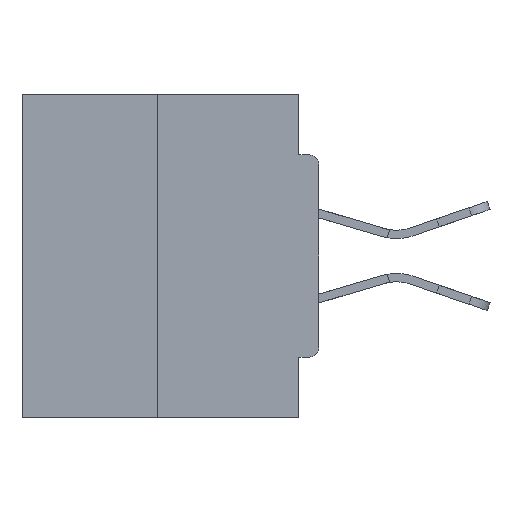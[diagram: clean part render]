
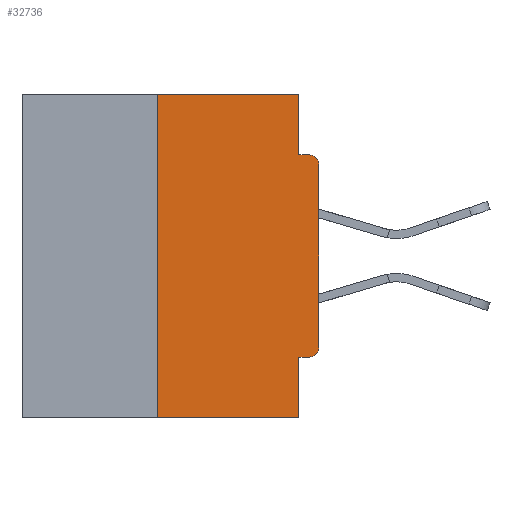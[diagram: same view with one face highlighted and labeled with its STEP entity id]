
A CAD part, left-side view. The second image highlights one B-rep face of the part: STEP entity #32736.
In plain terms, the highlighted planar face has unit normal (-1, 0, 0).
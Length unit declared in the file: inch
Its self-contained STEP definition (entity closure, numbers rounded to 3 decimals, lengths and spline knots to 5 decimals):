
#565 = CARTESIAN_POINT ( 'NONE',  ( 0., 0.25, 0. ) ) ;
#1227 = LINE ( 'NONE', #565, #5970 ) ;
#1453 = CARTESIAN_POINT ( 'NONE',  ( 0., 0.031, -0.0935 ) ) ;
#1588 = DIRECTION ( 'NONE',  ( -1., 0., 0. ) ) ;
#1603 = CARTESIAN_POINT ( 'NONE',  ( 0., 0., -0.3915 ) ) ;
#2099 = CARTESIAN_POINT ( 'NONE',  ( 0., 0.015, -0.0935 ) ) ;
#2642 = CARTESIAN_POINT ( 'NONE',  ( 0., 0., -0.4065 ) ) ;
#2885 = DIRECTION ( 'NONE',  ( 0., 1., 0. ) ) ;
#3850 = DIRECTION ( 'NONE',  ( 0., -1., 0. ) ) ;
#4548 = DIRECTION ( 'NONE',  ( -1., 0., 0. ) ) ;
#5272 = EDGE_CURVE ( 'NONE', #11194, #31900, #14237, .T. ) ;
#5275 = LINE ( 'NONE', #2642, #33623 ) ;
#5970 = VECTOR ( 'NONE', #25760, 39.37008 ) ;
#6230 = EDGE_CURVE ( 'NONE', #16097, #21846, #12427, .T. ) ;
#6483 = EDGE_CURVE ( 'NONE', #30119, #7789, #28742, .T. ) ;
#6925 = VECTOR ( 'NONE', #12689, 39.37008 ) ;
#7132 = LINE ( 'NONE', #23174, #15722 ) ;
#7213 = CARTESIAN_POINT ( 'NONE',  ( 0., 0.46, 0. ) ) ;
#7335 = DIRECTION ( 'NONE',  ( 0., 0., -1. ) ) ;
#7745 = ORIENTED_EDGE ( 'NONE', *, *, #12949, .F. ) ;
#7789 = VERTEX_POINT ( 'NONE', #22108 ) ;
#7847 = DIRECTION ( 'NONE',  ( 0., 0., 1. ) ) ;
#8564 = VECTOR ( 'NONE', #11351, 39.37008 ) ;
#8926 = CARTESIAN_POINT ( 'NONE',  ( 0., 0.46, 0. ) ) ;
#10336 = EDGE_CURVE ( 'NONE', #16097, #30119, #5275, .T. ) ;
#11194 = VERTEX_POINT ( 'NONE', #1453 ) ;
#11351 = DIRECTION ( 'NONE',  ( 0., 0., -1. ) ) ;
#12427 = CIRCLE ( 'NONE', #19663, 0.015 ) ;
#12654 = CARTESIAN_POINT ( 'NONE',  ( 0., 0.015, -0.1085 ) ) ;
#12689 = DIRECTION ( 'NONE',  ( 0., -1., 0. ) ) ;
#12803 = CARTESIAN_POINT ( 'NONE',  ( 0., 0., -0.0935 ) ) ;
#12949 = EDGE_CURVE ( 'NONE', #30383, #27522, #1227, .T. ) ;
#13443 = DIRECTION ( 'NONE',  ( 0., 0., -1. ) ) ;
#13752 = FACE_OUTER_BOUND ( 'NONE', #21500, .T. ) ;
#14123 = ORIENTED_EDGE ( 'NONE', *, *, #6230, .T. ) ;
#14237 = LINE ( 'NONE', #12803, #6925 ) ;
#15300 = AXIS2_PLACEMENT_3D ( 'NONE', #7213, #30117, #13443 ) ;
#15600 = PLANE ( 'NONE',  #15300 ) ;
#15700 = VECTOR ( 'NONE', #3850, 39.37008 ) ;
#15722 = VECTOR ( 'NONE', #26147, 39.37008 ) ;
#16097 = VERTEX_POINT ( 'NONE', #19459 ) ;
#16236 = LINE ( 'NONE', #16379, #34227 ) ;
#16379 = CARTESIAN_POINT ( 'NONE',  ( 0., 0., 0. ) ) ;
#18480 = CARTESIAN_POINT ( 'NONE',  ( 0., 0.25, -0.5 ) ) ;
#19179 = ORIENTED_EDGE ( 'NONE', *, *, #22291, .F. ) ;
#19270 = VECTOR ( 'NONE', #28973, 39.37008 ) ;
#19459 = CARTESIAN_POINT ( 'NONE',  ( 0., 0.015, -0.4065 ) ) ;
#19663 = AXIS2_PLACEMENT_3D ( 'NONE', #29741, #4548, #7335 ) ;
#19878 = EDGE_CURVE ( 'NONE', #21846, #28154, #16236, .T. ) ;
#20818 = DIRECTION ( 'NONE',  ( 0., 0., -1. ) ) ;
#21449 = EDGE_CURVE ( 'NONE', #35226, #11194, #7132, .T. ) ;
#21500 = EDGE_LOOP ( 'NONE', ( #19179, #7745, #25958, #30242, #27048, #14123, #27837, #33253, #30404, #28210 ) ) ;
#21846 = VERTEX_POINT ( 'NONE', #1603 ) ;
#22108 = CARTESIAN_POINT ( 'NONE',  ( 0., 0.031, -0.5 ) ) ;
#22276 = CARTESIAN_POINT ( 'NONE',  ( 0., 0.031, -0.5 ) ) ;
#22291 = EDGE_CURVE ( 'NONE', #27522, #35226, #30291, .T. ) ;
#22928 = CARTESIAN_POINT ( 'NONE',  ( 0., 0.031, -0.4065 ) ) ;
#23174 = CARTESIAN_POINT ( 'NONE',  ( 0., 0.031, 0. ) ) ;
#24320 = AXIS2_PLACEMENT_3D ( 'NONE', #12654, #1588, #20818 ) ;
#25141 = CARTESIAN_POINT ( 'NONE',  ( 0., 0.25, 0. ) ) ;
#25715 = LINE ( 'NONE', #34210, #19270 ) ;
#25760 = DIRECTION ( 'NONE',  ( 0., 0., 1. ) ) ;
#25958 = ORIENTED_EDGE ( 'NONE', *, *, #34543, .T. ) ;
#26147 = DIRECTION ( 'NONE',  ( 0., 0., -1. ) ) ;
#27048 = ORIENTED_EDGE ( 'NONE', *, *, #10336, .F. ) ;
#27522 = VERTEX_POINT ( 'NONE', #25141 ) ;
#27837 = ORIENTED_EDGE ( 'NONE', *, *, #19878, .T. ) ;
#28154 = VERTEX_POINT ( 'NONE', #34078 ) ;
#28210 = ORIENTED_EDGE ( 'NONE', *, *, #21449, .F. ) ;
#28742 = LINE ( 'NONE', #22276, #8564 ) ;
#28973 = DIRECTION ( 'NONE',  ( 0., -1., 0. ) ) ;
#29399 = CARTESIAN_POINT ( 'NONE',  ( 0., 0.031, 0. ) ) ;
#29741 = CARTESIAN_POINT ( 'NONE',  ( 0., 0.015, -0.3915 ) ) ;
#30117 = DIRECTION ( 'NONE',  ( 1., 0., 0. ) ) ;
#30119 = VERTEX_POINT ( 'NONE', #22928 ) ;
#30242 = ORIENTED_EDGE ( 'NONE', *, *, #6483, .F. ) ;
#30291 = LINE ( 'NONE', #8926, #15700 ) ;
#30383 = VERTEX_POINT ( 'NONE', #18480 ) ;
#30404 = ORIENTED_EDGE ( 'NONE', *, *, #5272, .F. ) ;
#31330 = EDGE_CURVE ( 'NONE', #28154, #31900, #31606, .T. ) ;
#31606 = CIRCLE ( 'NONE', #24320, 0.015 ) ;
#31900 = VERTEX_POINT ( 'NONE', #2099 ) ;
#32736 = ADVANCED_FACE ( 'NONE', ( #13752 ), #15600, .F. ) ;
#33253 = ORIENTED_EDGE ( 'NONE', *, *, #31330, .T. ) ;
#33623 = VECTOR ( 'NONE', #2885, 39.37008 ) ;
#34078 = CARTESIAN_POINT ( 'NONE',  ( 0., 0., -0.1085 ) ) ;
#34210 = CARTESIAN_POINT ( 'NONE',  ( 0., 0.46, -0.5 ) ) ;
#34227 = VECTOR ( 'NONE', #7847, 39.37008 ) ;
#34543 = EDGE_CURVE ( 'NONE', #30383, #7789, #25715, .T. ) ;
#35226 = VERTEX_POINT ( 'NONE', #29399 ) ;
